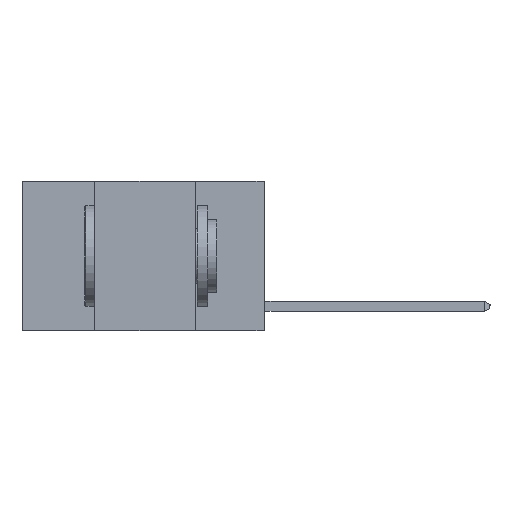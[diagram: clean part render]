
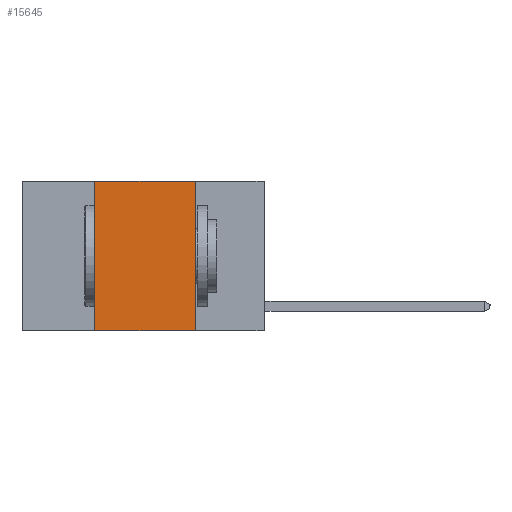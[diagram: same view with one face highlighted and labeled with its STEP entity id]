
A CAD part, left-side view. The second image highlights one B-rep face of the part: STEP entity #15645.
In plain terms, the highlighted planar face has unit normal (-1, 0, 0).
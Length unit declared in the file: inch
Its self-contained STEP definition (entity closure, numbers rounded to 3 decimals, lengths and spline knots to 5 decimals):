
#143 = ORIENTED_EDGE ( 'NONE', *, *, #13094, .T. ) ;
#621 = CARTESIAN_POINT ( 'NONE',  ( 0., 0.6, -0.37 ) ) ;
#629 = CARTESIAN_POINT ( 'NONE',  ( 0., 0.6, 0. ) ) ;
#1547 = VERTEX_POINT ( 'NONE', #8234 ) ;
#1721 = LINE ( 'NONE', #5869, #9076 ) ;
#3025 = CARTESIAN_POINT ( 'NONE',  ( 0., 0.42, 0. ) ) ;
#3287 = CARTESIAN_POINT ( 'NONE',  ( 0., 0.17, 0. ) ) ;
#3294 = DIRECTION ( 'NONE',  ( 0., 0., -1. ) ) ;
#3374 = EDGE_CURVE ( 'NONE', #9017, #13095, #6830, .T. ) ;
#3377 = VECTOR ( 'NONE', #5459, 39.37008 ) ;
#4846 = VECTOR ( 'NONE', #14429, 39.37008 ) ;
#5024 = ORIENTED_EDGE ( 'NONE', *, *, #15625, .F. ) ;
#5439 = CARTESIAN_POINT ( 'NONE',  ( 0., 0.6, 0. ) ) ;
#5459 = DIRECTION ( 'NONE',  ( 0., -1., 0. ) ) ;
#5795 = VECTOR ( 'NONE', #13540, 39.37008 ) ;
#5869 = CARTESIAN_POINT ( 'NONE',  ( 0., 0.42, 0. ) ) ;
#6830 = LINE ( 'NONE', #5439, #3377 ) ;
#8234 = CARTESIAN_POINT ( 'NONE',  ( 0., 0.17, -0.37 ) ) ;
#8460 = PLANE ( 'NONE',  #12755 ) ;
#8964 = ORIENTED_EDGE ( 'NONE', *, *, #14774, .F. ) ;
#9017 = VERTEX_POINT ( 'NONE', #3025 ) ;
#9076 = VECTOR ( 'NONE', #14801, 39.37008 ) ;
#9242 = LINE ( 'NONE', #621, #5795 ) ;
#9987 = EDGE_LOOP ( 'NONE', ( #8964, #15908, #5024, #143 ) ) ;
#10687 = CARTESIAN_POINT ( 'NONE',  ( 0., 0.17, 0. ) ) ;
#11072 = DIRECTION ( 'NONE',  ( 1., 0., 0. ) ) ;
#11443 = VERTEX_POINT ( 'NONE', #14192 ) ;
#12108 = LINE ( 'NONE', #10687, #4846 ) ;
#12755 = AXIS2_PLACEMENT_3D ( 'NONE', #629, #11072, #3294 ) ;
#13094 = EDGE_CURVE ( 'NONE', #11443, #1547, #9242, .T. ) ;
#13095 = VERTEX_POINT ( 'NONE', #3287 ) ;
#13540 = DIRECTION ( 'NONE',  ( 0., -1., 0. ) ) ;
#14192 = CARTESIAN_POINT ( 'NONE',  ( 0., 0.42, -0.37 ) ) ;
#14429 = DIRECTION ( 'NONE',  ( 0., 0., -1. ) ) ;
#14774 = EDGE_CURVE ( 'NONE', #13095, #1547, #12108, .T. ) ;
#14801 = DIRECTION ( 'NONE',  ( 0., 0., 1. ) ) ;
#15035 = FACE_OUTER_BOUND ( 'NONE', #9987, .T. ) ;
#15625 = EDGE_CURVE ( 'NONE', #11443, #9017, #1721, .T. ) ;
#15645 = ADVANCED_FACE ( 'NONE', ( #15035 ), #8460, .F. ) ;
#15908 = ORIENTED_EDGE ( 'NONE', *, *, #3374, .F. ) ;
